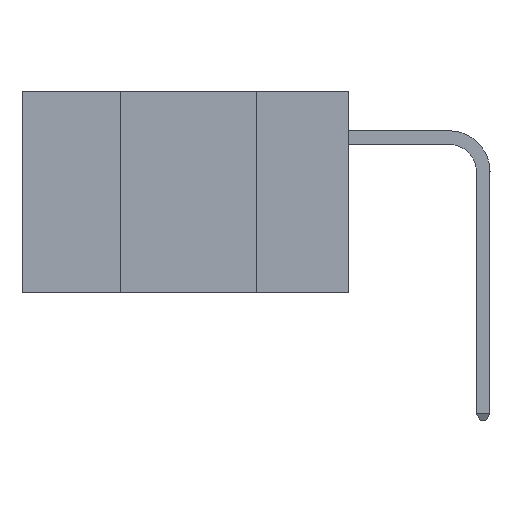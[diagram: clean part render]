
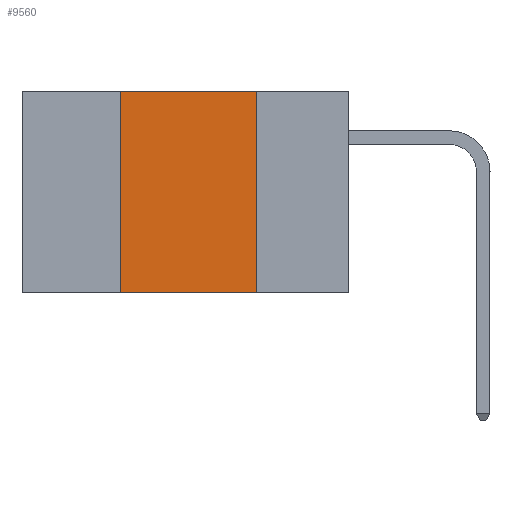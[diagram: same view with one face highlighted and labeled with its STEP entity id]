
A CAD part, left-side view. The second image highlights one B-rep face of the part: STEP entity #9560.
In plain terms, the highlighted planar face has unit normal (-1, 0, 0).
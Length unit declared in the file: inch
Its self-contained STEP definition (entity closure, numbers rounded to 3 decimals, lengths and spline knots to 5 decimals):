
#1641 = CARTESIAN_POINT ( 'NONE',  ( 0., 0.42, 0. ) ) ;
#2049 = VERTEX_POINT ( 'NONE', #27800 ) ;
#2612 = CARTESIAN_POINT ( 'NONE',  ( 0., 0.6, 0. ) ) ;
#5182 = CARTESIAN_POINT ( 'NONE',  ( 0., 0.17, 0. ) ) ;
#5710 = CARTESIAN_POINT ( 'NONE',  ( 0., 0.6, -0.37 ) ) ;
#7339 = LINE ( 'NONE', #11368, #22952 ) ;
#8927 = DIRECTION ( 'NONE',  ( 0., -1., 0. ) ) ;
#9560 = ADVANCED_FACE ( 'NONE', ( #17121 ), #30682, .F. ) ;
#9568 = LINE ( 'NONE', #5710, #38365 ) ;
#10137 = ORIENTED_EDGE ( 'NONE', *, *, #27318, .F. ) ;
#10166 = VECTOR ( 'NONE', #33100, 39.37008 ) ;
#11368 = CARTESIAN_POINT ( 'NONE',  ( 0., 0.42, 0. ) ) ;
#12280 = CARTESIAN_POINT ( 'NONE',  ( 0., 0.6, 0. ) ) ;
#12774 = LINE ( 'NONE', #12280, #28125 ) ;
#13071 = VERTEX_POINT ( 'NONE', #23922 ) ;
#13164 = ORIENTED_EDGE ( 'NONE', *, *, #34661, .F. ) ;
#14058 = ORIENTED_EDGE ( 'NONE', *, *, #38205, .T. ) ;
#14540 = DIRECTION ( 'NONE',  ( 0., 0., 1. ) ) ;
#15447 = DIRECTION ( 'NONE',  ( 0., -1., 0. ) ) ;
#15475 = DIRECTION ( 'NONE',  ( 0., 0., -1. ) ) ;
#16427 = VERTEX_POINT ( 'NONE', #1641 ) ;
#17121 = FACE_OUTER_BOUND ( 'NONE', #29454, .T. ) ;
#19643 = EDGE_CURVE ( 'NONE', #13071, #28438, #33728, .T. ) ;
#22952 = VECTOR ( 'NONE', #14540, 39.37008 ) ;
#23922 = CARTESIAN_POINT ( 'NONE',  ( 0., 0.17, 0. ) ) ;
#27318 = EDGE_CURVE ( 'NONE', #16427, #13071, #12774, .T. ) ;
#27510 = ORIENTED_EDGE ( 'NONE', *, *, #19643, .F. ) ;
#27800 = CARTESIAN_POINT ( 'NONE',  ( 0., 0.42, -0.37 ) ) ;
#28125 = VECTOR ( 'NONE', #15447, 39.37008 ) ;
#28294 = CARTESIAN_POINT ( 'NONE',  ( 0., 0.17, -0.37 ) ) ;
#28438 = VERTEX_POINT ( 'NONE', #28294 ) ;
#29454 = EDGE_LOOP ( 'NONE', ( #27510, #10137, #13164, #14058 ) ) ;
#30682 = PLANE ( 'NONE',  #32576 ) ;
#32576 = AXIS2_PLACEMENT_3D ( 'NONE', #2612, #33725, #15475 ) ;
#33100 = DIRECTION ( 'NONE',  ( 0., 0., -1. ) ) ;
#33725 = DIRECTION ( 'NONE',  ( 1., 0., 0. ) ) ;
#33728 = LINE ( 'NONE', #5182, #10166 ) ;
#34661 = EDGE_CURVE ( 'NONE', #2049, #16427, #7339, .T. ) ;
#38205 = EDGE_CURVE ( 'NONE', #2049, #28438, #9568, .T. ) ;
#38365 = VECTOR ( 'NONE', #8927, 39.37008 ) ;
